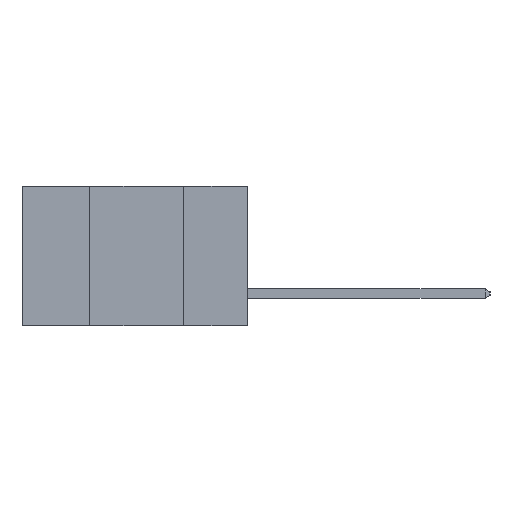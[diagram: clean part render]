
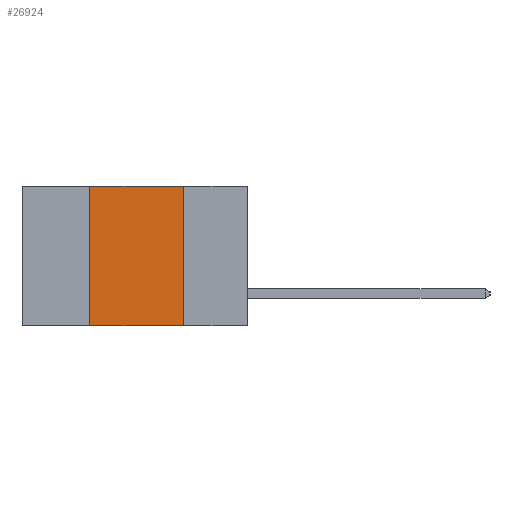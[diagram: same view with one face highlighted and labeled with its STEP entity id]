
A CAD part, left-side view. The second image highlights one B-rep face of the part: STEP entity #26924.
In plain terms, the highlighted planar face has unit normal (-1, 0, 0).
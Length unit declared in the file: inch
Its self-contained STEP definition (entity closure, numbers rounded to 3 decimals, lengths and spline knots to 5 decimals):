
#107 = DIRECTION ( 'NONE',  ( 0., 0., -1. ) ) ;
#876 = EDGE_CURVE ( 'NONE', #27658, #14249, #23802, .T. ) ;
#1561 = ORIENTED_EDGE ( 'NONE', *, *, #16091, .F. ) ;
#3081 = CARTESIAN_POINT ( 'NONE',  ( 0., 0.42, -0.37 ) ) ;
#3892 = EDGE_CURVE ( 'NONE', #26075, #27658, #12426, .T. ) ;
#5158 = EDGE_LOOP ( 'NONE', ( #27153, #6012, #1561, #20368 ) ) ;
#5193 = CARTESIAN_POINT ( 'NONE',  ( 0., 0.17, 0. ) ) ;
#5244 = FACE_OUTER_BOUND ( 'NONE', #5158, .T. ) ;
#6012 = ORIENTED_EDGE ( 'NONE', *, *, #3892, .F. ) ;
#6088 = AXIS2_PLACEMENT_3D ( 'NONE', #26283, #13237, #107 ) ;
#6620 = VECTOR ( 'NONE', #9810, 39.37008 ) ;
#7935 = DIRECTION ( 'NONE',  ( 0., 0., 1. ) ) ;
#8296 = DIRECTION ( 'NONE',  ( 0., -1., 0. ) ) ;
#8889 = LINE ( 'NONE', #21357, #26270 ) ;
#9810 = DIRECTION ( 'NONE',  ( 0., -1., 0. ) ) ;
#10011 = CARTESIAN_POINT ( 'NONE',  ( 0., 0.6, 0. ) ) ;
#10221 = EDGE_CURVE ( 'NONE', #24367, #14249, #8889, .T. ) ;
#10235 = LINE ( 'NONE', #25255, #26951 ) ;
#10422 = DIRECTION ( 'NONE',  ( 0., 0., -1. ) ) ;
#10457 = CARTESIAN_POINT ( 'NONE',  ( 0., 0.17, 0. ) ) ;
#12233 = VECTOR ( 'NONE', #10422, 39.37008 ) ;
#12426 = LINE ( 'NONE', #10011, #6620 ) ;
#13237 = DIRECTION ( 'NONE',  ( 1., 0., 0. ) ) ;
#14249 = VERTEX_POINT ( 'NONE', #23641 ) ;
#16091 = EDGE_CURVE ( 'NONE', #24367, #26075, #10235, .T. ) ;
#20368 = ORIENTED_EDGE ( 'NONE', *, *, #10221, .T. ) ;
#21357 = CARTESIAN_POINT ( 'NONE',  ( 0., 0.6, -0.37 ) ) ;
#23641 = CARTESIAN_POINT ( 'NONE',  ( 0., 0.17, -0.37 ) ) ;
#23802 = LINE ( 'NONE', #10457, #12233 ) ;
#24244 = CARTESIAN_POINT ( 'NONE',  ( 0., 0.42, 0. ) ) ;
#24367 = VERTEX_POINT ( 'NONE', #3081 ) ;
#25255 = CARTESIAN_POINT ( 'NONE',  ( 0., 0.42, 0. ) ) ;
#26075 = VERTEX_POINT ( 'NONE', #24244 ) ;
#26193 = PLANE ( 'NONE',  #6088 ) ;
#26270 = VECTOR ( 'NONE', #8296, 39.37008 ) ;
#26283 = CARTESIAN_POINT ( 'NONE',  ( 0., 0.6, 0. ) ) ;
#26924 = ADVANCED_FACE ( 'NONE', ( #5244 ), #26193, .F. ) ;
#26951 = VECTOR ( 'NONE', #7935, 39.37008 ) ;
#27153 = ORIENTED_EDGE ( 'NONE', *, *, #876, .F. ) ;
#27658 = VERTEX_POINT ( 'NONE', #5193 ) ;
